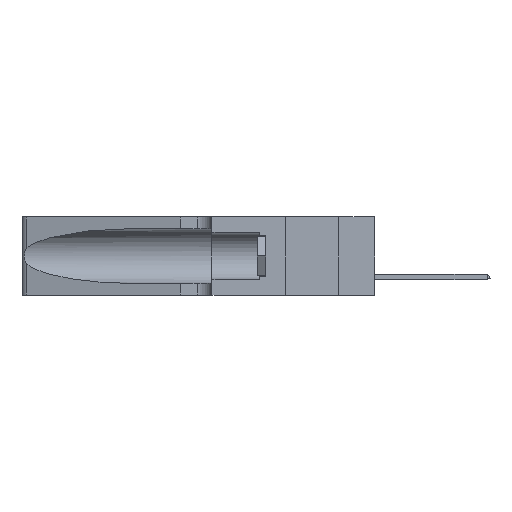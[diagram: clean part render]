
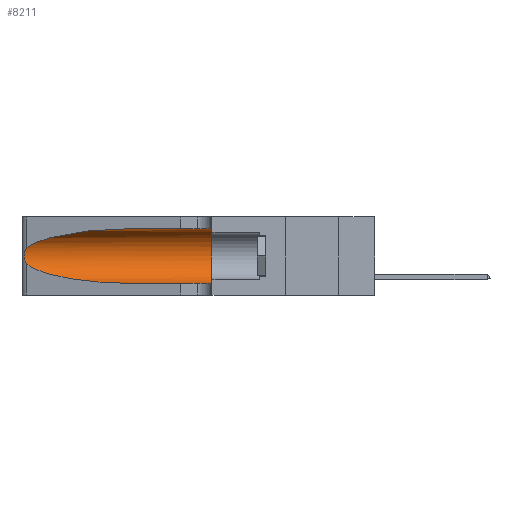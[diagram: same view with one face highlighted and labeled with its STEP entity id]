
A CAD part, left-side view. The second image highlights one B-rep face of the part: STEP entity #8211.
In plain terms, the highlighted cylindrical face has radius 3.308 mm (diameter 6.617 mm), a partial arc.
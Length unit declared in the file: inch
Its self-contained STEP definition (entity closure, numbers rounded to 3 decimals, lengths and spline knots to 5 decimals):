
#257 = DIRECTION ( 'NONE',  ( 0., -1., 0. ) ) ;
#339 = VERTEX_POINT ( 'NONE', #21062 ) ;
#856 = CIRCLE ( 'NONE', #20340, 0.13025 ) ;
#2323 =( BOUNDED_CURVE ( )  B_SPLINE_CURVE ( 3, ( #34400, #7993, #23099, #19929 ),
 .UNSPECIFIED., .F., .F. ) 
 B_SPLINE_CURVE_WITH_KNOTS ( ( 4, 4 ),
 ( 1.5708, 2.84003 ),
 .UNSPECIFIED. ) 
 CURVE ( )  GEOMETRIC_REPRESENTATION_ITEM ( )  RATIONAL_B_SPLINE_CURVE ( ( 1., 0.87, 0.87, 1. ) ) 
 REPRESENTATION_ITEM ( '' )  );
#3125 = EDGE_LOOP ( 'NONE', ( #18320, #32196, #32508, #32130, #9132, #36715 ) ) ;
#3991 = CARTESIAN_POINT ( 'NONE',  ( 0.1305, 1.61858, 0.31525 ) ) ;
#4223 = CARTESIAN_POINT ( 'NONE',  ( 0.1305, 0.35, 0.05475 ) ) ;
#5676 = CARTESIAN_POINT ( 'NONE',  ( 0.1305, 0.35, 0.185 ) ) ;
#6169 = CARTESIAN_POINT ( 'NONE',  ( 0.1305, 1.61858, 0.05475 ) ) ;
#6295 = VERTEX_POINT ( 'NONE', #6659 ) ;
#6659 = CARTESIAN_POINT ( 'NONE',  ( 0.1305, 0.72297, 0.31525 ) ) ;
#7267 = CARTESIAN_POINT ( 'NONE',  ( 0.25487, 1.22718, 0.14631 ) ) ;
#7993 = CARTESIAN_POINT ( 'NONE',  ( 0.18966, 0.96281, 0.31525 ) ) ;
#8191 = CARTESIAN_POINT ( 'NONE',  ( 0.25487, 1.22718, 0.14631 ) ) ;
#8211 = ADVANCED_FACE ( 'NONE', ( #11166 ), #25249, .F. ) ;
#8611 = CARTESIAN_POINT ( 'NONE',  ( 0.26075, 1.23896, 0.178 ) ) ;
#9030 = CARTESIAN_POINT ( 'NONE',  ( 0.2373, 1.15595, 0.08982 ) ) ;
#9032 =( BOUNDED_CURVE ( )  B_SPLINE_CURVE ( 3, ( #7267, #9030, #31517, #14088 ),
 .UNSPECIFIED., .F., .F. ) 
 B_SPLINE_CURVE_WITH_KNOTS ( ( 4, 4 ),
 ( 3.44316, 4.71239 ),
 .UNSPECIFIED. ) 
 CURVE ( )  GEOMETRIC_REPRESENTATION_ITEM ( )  RATIONAL_B_SPLINE_CURVE ( ( 1., 0.87, 0.87, 1. ) ) 
 REPRESENTATION_ITEM ( '' )  );
#9132 = ORIENTED_EDGE ( 'NONE', *, *, #11535, .F. ) ;
#9189 = VECTOR ( 'NONE', #26992, 39.37008 ) ;
#9647 = EDGE_CURVE ( 'NONE', #6295, #35937, #33741, .T. ) ;
#11166 = FACE_OUTER_BOUND ( 'NONE', #3125, .T. ) ;
#11423 = CARTESIAN_POINT ( 'NONE',  ( 0.25487, 1.22718, 0.22369 ) ) ;
#11535 = EDGE_CURVE ( 'NONE', #35937, #26042, #856, .T. ) ;
#11538 = CARTESIAN_POINT ( 'NONE',  ( 0.25856, 1.23593, 0.16098 ) ) ;
#11750 = CARTESIAN_POINT ( 'NONE',  ( 0.25555, 1.22993, 0.14849 ) ) ;
#13961 = DIRECTION ( 'NONE',  ( 0., -1., 0. ) ) ;
#14088 = CARTESIAN_POINT ( 'NONE',  ( 0.1305, 0.72297, 0.05475 ) ) ;
#14661 = CARTESIAN_POINT ( 'NONE',  ( 0.25487, 1.22718, 0.14631 ) ) ;
#15114 = EDGE_CURVE ( 'NONE', #339, #26042, #22167, .T. ) ;
#18320 = ORIENTED_EDGE ( 'NONE', *, *, #29940, .T. ) ;
#19739 = EDGE_CURVE ( 'NONE', #34299, #28882, #23064, .T. ) ;
#19929 = CARTESIAN_POINT ( 'NONE',  ( 0.25487, 1.22718, 0.22369 ) ) ;
#20059 = CARTESIAN_POINT ( 'NONE',  ( 0.25787, 1.23484, 0.2124 ) ) ;
#20173 = CARTESIAN_POINT ( 'NONE',  ( 0.26075, 1.23896, 0.19203 ) ) ;
#20340 = AXIS2_PLACEMENT_3D ( 'NONE', #5676, #25922, #23717 ) ;
#21062 = CARTESIAN_POINT ( 'NONE',  ( 0.1305, 0.72297, 0.05475 ) ) ;
#22167 = LINE ( 'NONE', #6169, #33034 ) ;
#22864 = CARTESIAN_POINT ( 'NONE',  ( 0.25555, 1.22994, 0.2215 ) ) ;
#23064 = B_SPLINE_CURVE_WITH_KNOTS ( 'NONE', 3,
 ( #11423, #22864, #31742, #20059, #25915, #23107, #20173, #8611, #28932, #11538, #31864, #31984, #11750, #14661 ),
 .UNSPECIFIED., .F., .F.,
 ( 4, 2, 2, 2, 2, 2, 4 ),
 ( 0., 0.00027, 0.00053, 0.00107, 0.0016, 0.00187, 0.00214 ),
 .UNSPECIFIED. ) ;
#23070 = CARTESIAN_POINT ( 'NONE',  ( 0.25487, 1.22718, 0.22369 ) ) ;
#23099 = CARTESIAN_POINT ( 'NONE',  ( 0.2373, 1.15595, 0.28018 ) ) ;
#23107 = CARTESIAN_POINT ( 'NONE',  ( 0.26018, 1.23835, 0.19895 ) ) ;
#23178 = AXIS2_PLACEMENT_3D ( 'NONE', #31377, #13961, #25806 ) ;
#23717 = DIRECTION ( 'NONE',  ( 0., 0., 1. ) ) ;
#25249 = CYLINDRICAL_SURFACE ( 'NONE', #23178, 0.13025 ) ;
#25616 = EDGE_CURVE ( 'NONE', #28882, #339, #9032, .T. ) ;
#25806 = DIRECTION ( 'NONE',  ( 0., 0., -1. ) ) ;
#25915 = CARTESIAN_POINT ( 'NONE',  ( 0.25854, 1.2359, 0.20912 ) ) ;
#25922 = DIRECTION ( 'NONE',  ( 0., 1., 0. ) ) ;
#26042 = VERTEX_POINT ( 'NONE', #4223 ) ;
#26992 = DIRECTION ( 'NONE',  ( 0., -1., 0. ) ) ;
#28882 = VERTEX_POINT ( 'NONE', #8191 ) ;
#28932 = CARTESIAN_POINT ( 'NONE',  ( 0.26017, 1.23833, 0.17102 ) ) ;
#29940 = EDGE_CURVE ( 'NONE', #6295, #34299, #2323, .T. ) ;
#31377 = CARTESIAN_POINT ( 'NONE',  ( 0.1305, 1.61858, 0.185 ) ) ;
#31517 = CARTESIAN_POINT ( 'NONE',  ( 0.18966, 0.96281, 0.05475 ) ) ;
#31742 = CARTESIAN_POINT ( 'NONE',  ( 0.25639, 1.23184, 0.21858 ) ) ;
#31864 = CARTESIAN_POINT ( 'NONE',  ( 0.25789, 1.23486, 0.15765 ) ) ;
#31984 = CARTESIAN_POINT ( 'NONE',  ( 0.25639, 1.23186, 0.15144 ) ) ;
#32130 = ORIENTED_EDGE ( 'NONE', *, *, #15114, .T. ) ;
#32196 = ORIENTED_EDGE ( 'NONE', *, *, #19739, .T. ) ;
#32470 = CARTESIAN_POINT ( 'NONE',  ( 0.1305, 0.35, 0.31525 ) ) ;
#32508 = ORIENTED_EDGE ( 'NONE', *, *, #25616, .T. ) ;
#33034 = VECTOR ( 'NONE', #257, 39.37008 ) ;
#33741 = LINE ( 'NONE', #3991, #9189 ) ;
#34299 = VERTEX_POINT ( 'NONE', #23070 ) ;
#34400 = CARTESIAN_POINT ( 'NONE',  ( 0.1305, 0.72297, 0.31525 ) ) ;
#35937 = VERTEX_POINT ( 'NONE', #32470 ) ;
#36715 = ORIENTED_EDGE ( 'NONE', *, *, #9647, .F. ) ;
